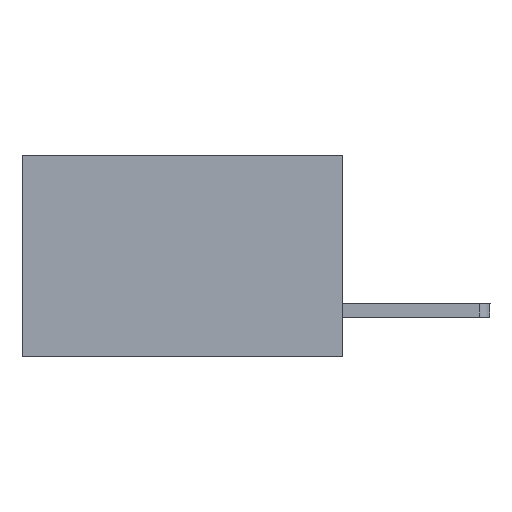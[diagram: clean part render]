
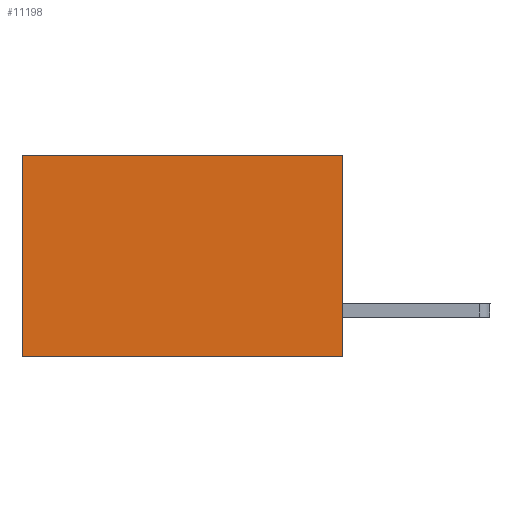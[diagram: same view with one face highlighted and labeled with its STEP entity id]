
A CAD part, left-side view. The second image highlights one B-rep face of the part: STEP entity #11198.
In plain terms, the highlighted planar face has unit normal (-1, 0, 0).
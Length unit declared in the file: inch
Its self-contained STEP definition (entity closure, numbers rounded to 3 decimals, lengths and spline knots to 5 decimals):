
#425 = VECTOR ( 'NONE', #2447, 39.37008 ) ;
#712 = CARTESIAN_POINT ( 'NONE',  ( 0.277, 0., 0. ) ) ;
#1455 = EDGE_CURVE ( 'NONE', #3776, #12502, #9760, .T. ) ;
#2447 = DIRECTION ( 'NONE',  ( 0., 1., 0. ) ) ;
#2515 = CARTESIAN_POINT ( 'NONE',  ( 0.277, 0., 0. ) ) ;
#2622 = DIRECTION ( 'NONE',  ( 0., 0., -1. ) ) ;
#2786 = LINE ( 'NONE', #3409, #5476 ) ;
#2929 = EDGE_LOOP ( 'NONE', ( #4945, #5436, #5660, #6317 ) ) ;
#3221 = CARTESIAN_POINT ( 'NONE',  ( 0.277, 0., -0.37 ) ) ;
#3409 = CARTESIAN_POINT ( 'NONE',  ( 0.277, 0., -0.37 ) ) ;
#3439 = DIRECTION ( 'NONE',  ( 0., 0., -1. ) ) ;
#3598 = DIRECTION ( 'NONE',  ( 1., 0., 0. ) ) ;
#3776 = VERTEX_POINT ( 'NONE', #9797 ) ;
#4097 = DIRECTION ( 'NONE',  ( 0., 1., 0. ) ) ;
#4372 = EDGE_CURVE ( 'NONE', #12025, #3776, #2786, .T. ) ;
#4943 = FACE_OUTER_BOUND ( 'NONE', #2929, .T. ) ;
#4945 = ORIENTED_EDGE ( 'NONE', *, *, #7429, .T. ) ;
#5436 = ORIENTED_EDGE ( 'NONE', *, *, #1455, .F. ) ;
#5476 = VECTOR ( 'NONE', #3439, 39.37008 ) ;
#5660 = ORIENTED_EDGE ( 'NONE', *, *, #4372, .F. ) ;
#6317 = ORIENTED_EDGE ( 'NONE', *, *, #6680, .T. ) ;
#6680 = EDGE_CURVE ( 'NONE', #12025, #6935, #9340, .T. ) ;
#6935 = VERTEX_POINT ( 'NONE', #9576 ) ;
#7429 = EDGE_CURVE ( 'NONE', #6935, #12502, #12261, .T. ) ;
#7601 = VECTOR ( 'NONE', #4097, 39.37008 ) ;
#9226 = CARTESIAN_POINT ( 'NONE',  ( 0.277, 0.59, -0.37 ) ) ;
#9340 = LINE ( 'NONE', #2515, #425 ) ;
#9576 = CARTESIAN_POINT ( 'NONE',  ( 0.277, 0.59, 0. ) ) ;
#9760 = LINE ( 'NONE', #3221, #7601 ) ;
#9797 = CARTESIAN_POINT ( 'NONE',  ( 0.277, 0., -0.37 ) ) ;
#9829 = VECTOR ( 'NONE', #2622, 39.37008 ) ;
#10003 = PLANE ( 'NONE',  #13718 ) ;
#10103 = CARTESIAN_POINT ( 'NONE',  ( 0.277, 0., -0.37 ) ) ;
#11168 = DIRECTION ( 'NONE',  ( 0., 0., -1. ) ) ;
#11198 = ADVANCED_FACE ( 'NONE', ( #4943 ), #10003, .F. ) ;
#12025 = VERTEX_POINT ( 'NONE', #712 ) ;
#12261 = LINE ( 'NONE', #9226, #9829 ) ;
#12353 = CARTESIAN_POINT ( 'NONE',  ( 0.277, 0.59, -0.37 ) ) ;
#12502 = VERTEX_POINT ( 'NONE', #12353 ) ;
#13718 = AXIS2_PLACEMENT_3D ( 'NONE', #10103, #3598, #11168 ) ;
